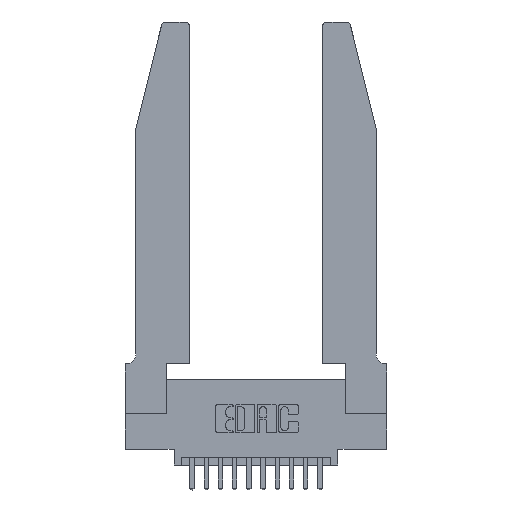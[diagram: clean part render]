
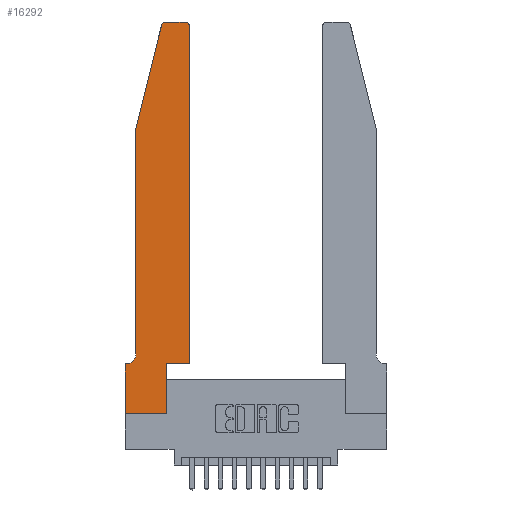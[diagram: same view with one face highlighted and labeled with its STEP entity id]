
A CAD part, top view. The second image highlights one B-rep face of the part: STEP entity #16292.
In plain terms, the highlighted planar face has unit normal (0, 0, 1).
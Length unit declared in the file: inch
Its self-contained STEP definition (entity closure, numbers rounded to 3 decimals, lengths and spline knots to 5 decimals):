
#79 = LINE ( 'NONE', #910, #12699 ) ;
#114 = EDGE_CURVE ( 'NONE', #5656, #2289, #15114, .T. ) ;
#153 = DIRECTION ( 'NONE',  ( 0., 1., 0. ) ) ;
#910 = CARTESIAN_POINT ( 'NONE',  ( 0.4505, 0.35, 0.37 ) ) ;
#1109 = CARTESIAN_POINT ( 'NONE',  ( 0.284, 2.72, 0.37 ) ) ;
#1449 = AXIS2_PLACEMENT_3D ( 'NONE', #15360, #8703, #2063 ) ;
#1877 = AXIS2_PLACEMENT_3D ( 'NONE', #13360, #7950, #4470 ) ;
#1921 = ORIENTED_EDGE ( 'NONE', *, *, #8848, .T. ) ;
#1952 = AXIS2_PLACEMENT_3D ( 'NONE', #16388, #8454, #11056 ) ;
#2063 = DIRECTION ( 'NONE',  ( 1., 0., 0. ) ) ;
#2289 = VERTEX_POINT ( 'NONE', #2767 ) ;
#2359 = CIRCLE ( 'NONE', #1952, 0.03 ) ;
#2423 = CARTESIAN_POINT ( 'NONE',  ( 0.4505, 2.72, 0.37 ) ) ;
#2528 = CARTESIAN_POINT ( 'NONE',  ( 0., 0., 0.37 ) ) ;
#2648 = EDGE_CURVE ( 'NONE', #14798, #13777, #5244, .T. ) ;
#2767 = CARTESIAN_POINT ( 'NONE',  ( 0.0055, 0.35, 0.37 ) ) ;
#2775 = VERTEX_POINT ( 'NONE', #16808 ) ;
#2789 = ORIENTED_EDGE ( 'NONE', *, *, #6599, .T. ) ;
#3000 = ORIENTED_EDGE ( 'NONE', *, *, #13210, .T. ) ;
#3034 = CARTESIAN_POINT ( 'NONE',  ( 0.2865, 0.35, 0.37 ) ) ;
#3144 = DIRECTION ( 'NONE',  ( 1., 0., 0. ) ) ;
#3179 = CARTESIAN_POINT ( 'NONE',  ( 0.0755, 2., 0.37 ) ) ;
#3243 = ORIENTED_EDGE ( 'NONE', *, *, #9245, .T. ) ;
#3513 = CARTESIAN_POINT ( 'NONE',  ( 0., 0.35, 0.37 ) ) ;
#3535 = FACE_OUTER_BOUND ( 'NONE', #11814, .T. ) ;
#3792 = CARTESIAN_POINT ( 'NONE',  ( 0.4205, 2.75, 0.37 ) ) ;
#4105 = EDGE_CURVE ( 'NONE', #13777, #10570, #7304, .T. ) ;
#4216 = DIRECTION ( 'NONE',  ( 0., -1., 0. ) ) ;
#4331 = EDGE_CURVE ( 'NONE', #11829, #16465, #12419, .T. ) ;
#4470 = DIRECTION ( 'NONE',  ( -1., 0., 0. ) ) ;
#4522 = DIRECTION ( 'NONE',  ( -1., 0., 0. ) ) ;
#4836 = PLANE ( 'NONE',  #1449 ) ;
#4877 = VERTEX_POINT ( 'NONE', #7015 ) ;
#4879 = EDGE_CURVE ( 'NONE', #2775, #9081, #14076, .T. ) ;
#5244 = LINE ( 'NONE', #5929, #17054 ) ;
#5289 = LINE ( 'NONE', #3034, #10465 ) ;
#5325 = VERTEX_POINT ( 'NONE', #3513 ) ;
#5467 = ORIENTED_EDGE ( 'NONE', *, *, #4331, .T. ) ;
#5470 = ORIENTED_EDGE ( 'NONE', *, *, #13158, .T. ) ;
#5571 = CARTESIAN_POINT ( 'NONE',  ( 0.0755, 2., 0.37 ) ) ;
#5656 = VERTEX_POINT ( 'NONE', #8417 ) ;
#5929 = CARTESIAN_POINT ( 'NONE',  ( 0.2605, 2.75, 0.37 ) ) ;
#6599 = EDGE_CURVE ( 'NONE', #2289, #5325, #7225, .T. ) ;
#6671 = DIRECTION ( 'NONE',  ( 0., -1., 0. ) ) ;
#6807 = CARTESIAN_POINT ( 'NONE',  ( 0.284, 2.75, 0.37 ) ) ;
#6870 = EDGE_CURVE ( 'NONE', #14968, #5656, #8858, .T. ) ;
#6877 = LINE ( 'NONE', #3179, #15983 ) ;
#6930 = CARTESIAN_POINT ( 'NONE',  ( 0.25487, 2.72718, 0.37 ) ) ;
#7015 = CARTESIAN_POINT ( 'NONE',  ( 0.2865, 0.35, 0.37 ) ) ;
#7225 = LINE ( 'NONE', #10954, #9674 ) ;
#7304 = CIRCLE ( 'NONE', #11347, 0.03 ) ;
#7555 = ORIENTED_EDGE ( 'NONE', *, *, #6870, .T. ) ;
#7950 = DIRECTION ( 'NONE',  ( 0., 0., -1. ) ) ;
#8380 = EDGE_CURVE ( 'NONE', #16465, #14798, #2359, .T. ) ;
#8417 = CARTESIAN_POINT ( 'NONE',  ( 0.0755, 0.42, 0.37 ) ) ;
#8454 = DIRECTION ( 'NONE',  ( 0., 0., 1. ) ) ;
#8703 = DIRECTION ( 'NONE',  ( 0., 0., 1. ) ) ;
#8848 = EDGE_CURVE ( 'NONE', #4877, #11829, #79, .T. ) ;
#8858 = LINE ( 'NONE', #15824, #11925 ) ;
#9081 = VERTEX_POINT ( 'NONE', #14948 ) ;
#9131 = DIRECTION ( 'NONE',  ( 0., 0., 1. ) ) ;
#9245 = EDGE_CURVE ( 'NONE', #10570, #14968, #6877, .T. ) ;
#9613 = VECTOR ( 'NONE', #4216, 39.37008 ) ;
#9674 = VECTOR ( 'NONE', #12257, 39.37008 ) ;
#9706 = CARTESIAN_POINT ( 'NONE',  ( 0., 0., 0.37 ) ) ;
#9818 = LINE ( 'NONE', #9706, #9613 ) ;
#10465 = VECTOR ( 'NONE', #12107, 39.37008 ) ;
#10570 = VERTEX_POINT ( 'NONE', #6930 ) ;
#10585 = VECTOR ( 'NONE', #12844, 39.37008 ) ;
#10954 = CARTESIAN_POINT ( 'NONE',  ( 0.0755, 0.35, 0.37 ) ) ;
#11056 = DIRECTION ( 'NONE',  ( 1., 0., 0. ) ) ;
#11347 = AXIS2_PLACEMENT_3D ( 'NONE', #1109, #9131, #14330 ) ;
#11814 = EDGE_LOOP ( 'NONE', ( #15104, #14147, #3243, #7555, #15109, #2789, #3000, #13311, #5470, #1921, #5467, #16132 ) ) ;
#11829 = VERTEX_POINT ( 'NONE', #16850 ) ;
#11925 = VECTOR ( 'NONE', #6671, 39.37008 ) ;
#12107 = DIRECTION ( 'NONE',  ( 0., 1., 0. ) ) ;
#12257 = DIRECTION ( 'NONE',  ( -1., 0., 0. ) ) ;
#12419 = LINE ( 'NONE', #13333, #14530 ) ;
#12423 = DIRECTION ( 'NONE',  ( -0.239, -0.971, 0. ) ) ;
#12699 = VECTOR ( 'NONE', #3144, 39.37008 ) ;
#12844 = DIRECTION ( 'NONE',  ( 1., 0., 0. ) ) ;
#13158 = EDGE_CURVE ( 'NONE', #9081, #4877, #5289, .T. ) ;
#13210 = EDGE_CURVE ( 'NONE', #5325, #2775, #9818, .T. ) ;
#13311 = ORIENTED_EDGE ( 'NONE', *, *, #4879, .T. ) ;
#13333 = CARTESIAN_POINT ( 'NONE',  ( 0.4505, 0.35, 0.37 ) ) ;
#13360 = CARTESIAN_POINT ( 'NONE',  ( 0.0055, 0.42, 0.37 ) ) ;
#13777 = VERTEX_POINT ( 'NONE', #6807 ) ;
#14076 = LINE ( 'NONE', #2528, #10585 ) ;
#14147 = ORIENTED_EDGE ( 'NONE', *, *, #4105, .T. ) ;
#14330 = DIRECTION ( 'NONE',  ( 1., 0., 0. ) ) ;
#14530 = VECTOR ( 'NONE', #153, 39.37008 ) ;
#14798 = VERTEX_POINT ( 'NONE', #3792 ) ;
#14948 = CARTESIAN_POINT ( 'NONE',  ( 0.2865, 0., 0.37 ) ) ;
#14968 = VERTEX_POINT ( 'NONE', #5571 ) ;
#15104 = ORIENTED_EDGE ( 'NONE', *, *, #2648, .T. ) ;
#15109 = ORIENTED_EDGE ( 'NONE', *, *, #114, .T. ) ;
#15114 = CIRCLE ( 'NONE', #1877, 0.07 ) ;
#15360 = CARTESIAN_POINT ( 'NONE',  ( 0., 0.35, 0.37 ) ) ;
#15824 = CARTESIAN_POINT ( 'NONE',  ( 0.0755, 2., 0.37 ) ) ;
#15983 = VECTOR ( 'NONE', #12423, 39.37008 ) ;
#16132 = ORIENTED_EDGE ( 'NONE', *, *, #8380, .T. ) ;
#16292 = ADVANCED_FACE ( 'NONE', ( #3535 ), #4836, .T. ) ;
#16388 = CARTESIAN_POINT ( 'NONE',  ( 0.4205, 2.72, 0.37 ) ) ;
#16465 = VERTEX_POINT ( 'NONE', #2423 ) ;
#16808 = CARTESIAN_POINT ( 'NONE',  ( 0., 0., 0.37 ) ) ;
#16850 = CARTESIAN_POINT ( 'NONE',  ( 0.4505, 0.35, 0.37 ) ) ;
#17054 = VECTOR ( 'NONE', #4522, 39.37008 ) ;
